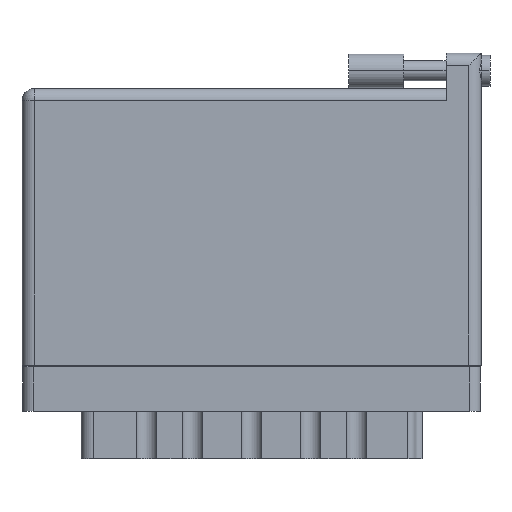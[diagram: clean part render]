
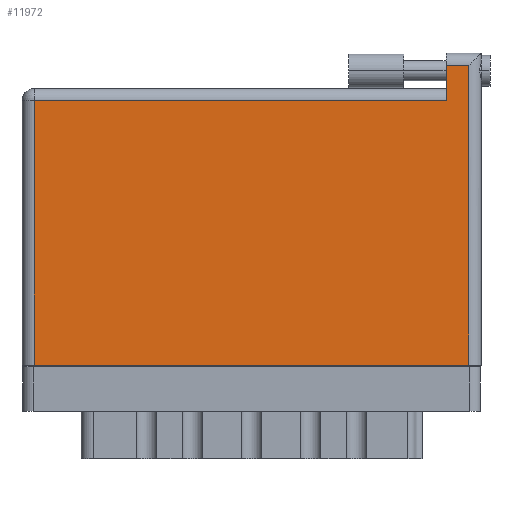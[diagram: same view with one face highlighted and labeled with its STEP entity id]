
A CAD part, front view. The second image highlights one B-rep face of the part: STEP entity #11972.
In plain terms, the highlighted face is planar.
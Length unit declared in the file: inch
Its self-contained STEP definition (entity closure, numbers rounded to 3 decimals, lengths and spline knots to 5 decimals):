
#1262 = EDGE_CURVE ( 'NONE', #34097, #6620, #6399, .T. ) ;
#2290 = ORIENTED_EDGE ( 'NONE', *, *, #2646, .T. ) ;
#2646 = EDGE_CURVE ( 'NONE', #35663, #7902, #25930, .T. ) ;
#4776 = LINE ( 'NONE', #10615, #37564 ) ;
#5378 = EDGE_CURVE ( 'NONE', #7902, #33336, #12672, .T. ) ;
#6040 = AXIS2_PLACEMENT_3D ( 'NONE', #40094, #36769, #21320 ) ;
#6122 = VECTOR ( 'NONE', #29368, 39.37008 ) ;
#6399 = LINE ( 'NONE', #19169, #24346 ) ;
#6620 = VERTEX_POINT ( 'NONE', #35377 ) ;
#7687 = EDGE_CURVE ( 'NONE', #21325, #34097, #4776, .T. ) ;
#7902 = VERTEX_POINT ( 'NONE', #30827 ) ;
#10136 = ORIENTED_EDGE ( 'NONE', *, *, #7687, .T. ) ;
#10615 = CARTESIAN_POINT ( 'NONE',  ( 0., 0., 0. ) ) ;
#10978 = EDGE_LOOP ( 'NONE', ( #10136, #27098, #22244, #2290, #46630, #29374 ) ) ;
#11972 = ADVANCED_FACE ( 'NONE', ( #45495 ), #36601, .F. ) ;
#12672 = LINE ( 'NONE', #13973, #6122 ) ;
#13973 = CARTESIAN_POINT ( 'NONE',  ( 0., 1.496, 0. ) ) ;
#16026 = LINE ( 'NONE', #16331, #16609 ) ;
#16331 = CARTESIAN_POINT ( 'NONE',  ( 0.07, 0., 0. ) ) ;
#16575 = CARTESIAN_POINT ( 'NONE',  ( 0.07, 0., 0. ) ) ;
#16609 = VECTOR ( 'NONE', #20180, 39.37008 ) ;
#18276 = CARTESIAN_POINT ( 'NONE',  ( 2.403, 1.766, 0. ) ) ;
#19169 = CARTESIAN_POINT ( 'NONE',  ( 2.53, 1.766, 0. ) ) ;
#20180 = DIRECTION ( 'NONE',  ( 0., -1., 0. ) ) ;
#20537 = VECTOR ( 'NONE', #44913, 39.37008 ) ;
#21320 = DIRECTION ( 'NONE',  ( -1., 0., 0. ) ) ;
#21325 = VERTEX_POINT ( 'NONE', #16575 ) ;
#22244 = ORIENTED_EDGE ( 'NONE', *, *, #40704, .T. ) ;
#24346 = VECTOR ( 'NONE', #34679, 39.37008 ) ;
#25382 = CARTESIAN_POINT ( 'NONE',  ( 0., 1.696, 0. ) ) ;
#25930 = LINE ( 'NONE', #18276, #20537 ) ;
#27098 = ORIENTED_EDGE ( 'NONE', *, *, #1262, .T. ) ;
#27182 = CARTESIAN_POINT ( 'NONE',  ( 2.403, 1.696, 0. ) ) ;
#28707 = DIRECTION ( 'NONE',  ( -1., 0., 0. ) ) ;
#29120 = CARTESIAN_POINT ( 'NONE',  ( 2.53, 0., 0. ) ) ;
#29368 = DIRECTION ( 'NONE',  ( -1., 0., 0. ) ) ;
#29374 = ORIENTED_EDGE ( 'NONE', *, *, #35129, .T. ) ;
#29690 = DIRECTION ( 'NONE',  ( 1., 0., 0. ) ) ;
#30827 = CARTESIAN_POINT ( 'NONE',  ( 2.403, 1.496, 0. ) ) ;
#32287 = LINE ( 'NONE', #25382, #42976 ) ;
#33336 = VERTEX_POINT ( 'NONE', #45616 ) ;
#34097 = VERTEX_POINT ( 'NONE', #29120 ) ;
#34679 = DIRECTION ( 'NONE',  ( 0., 1., 0. ) ) ;
#35129 = EDGE_CURVE ( 'NONE', #33336, #21325, #16026, .T. ) ;
#35377 = CARTESIAN_POINT ( 'NONE',  ( 2.53, 1.696, 0. ) ) ;
#35663 = VERTEX_POINT ( 'NONE', #27182 ) ;
#36601 = PLANE ( 'NONE',  #6040 ) ;
#36769 = DIRECTION ( 'NONE',  ( 0., 0., -1. ) ) ;
#37564 = VECTOR ( 'NONE', #29690, 39.37008 ) ;
#40094 = CARTESIAN_POINT ( 'NONE',  ( 0., 1.566, 0. ) ) ;
#40704 = EDGE_CURVE ( 'NONE', #6620, #35663, #32287, .T. ) ;
#42976 = VECTOR ( 'NONE', #28707, 39.37008 ) ;
#44913 = DIRECTION ( 'NONE',  ( 0., -1., 0. ) ) ;
#45495 = FACE_OUTER_BOUND ( 'NONE', #10978, .T. ) ;
#45616 = CARTESIAN_POINT ( 'NONE',  ( 0.07, 1.496, 0. ) ) ;
#46630 = ORIENTED_EDGE ( 'NONE', *, *, #5378, .T. ) ;
